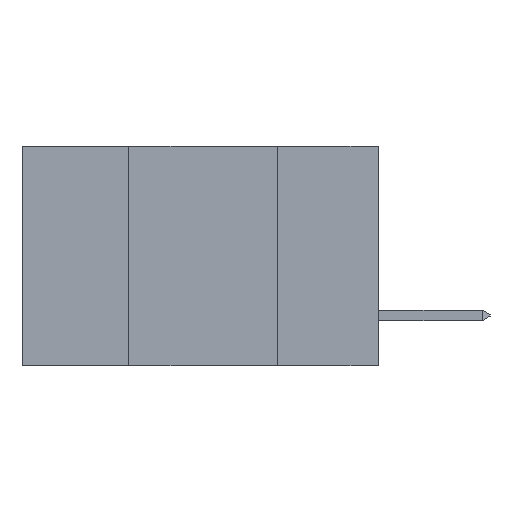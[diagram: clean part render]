
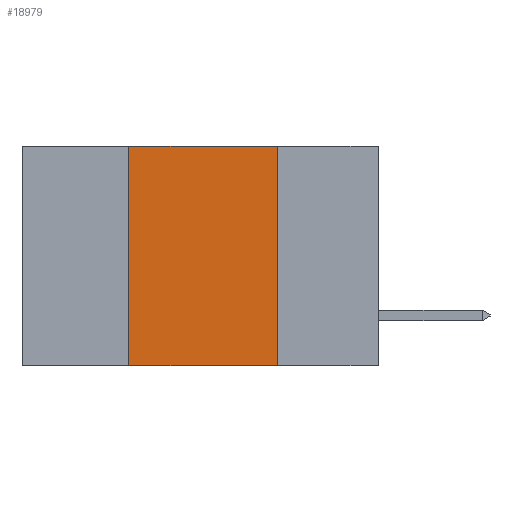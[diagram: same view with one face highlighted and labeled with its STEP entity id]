
A CAD part, left-side view. The second image highlights one B-rep face of the part: STEP entity #18979.
In plain terms, the highlighted planar face has unit normal (-1, 0, 0).
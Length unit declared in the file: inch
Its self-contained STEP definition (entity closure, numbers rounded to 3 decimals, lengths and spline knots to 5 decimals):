
#715 = EDGE_LOOP ( 'NONE', ( #17056, #18453, #7615, #10102 ) ) ;
#2209 = EDGE_CURVE ( 'NONE', #14121, #18918, #9257, .T. ) ;
#2323 = DIRECTION ( 'NONE',  ( 0., 0., -1. ) ) ;
#2471 = VERTEX_POINT ( 'NONE', #14462 ) ;
#2641 = LINE ( 'NONE', #3035, #10462 ) ;
#2938 = FACE_OUTER_BOUND ( 'NONE', #715, .T. ) ;
#3035 = CARTESIAN_POINT ( 'NONE',  ( 0., 0.42, 0. ) ) ;
#3859 = EDGE_CURVE ( 'NONE', #4077, #18918, #12831, .T. ) ;
#4077 = VERTEX_POINT ( 'NONE', #9818 ) ;
#4919 = DIRECTION ( 'NONE',  ( 0., -1., 0. ) ) ;
#5642 = EDGE_CURVE ( 'NONE', #2471, #4077, #7486, .T. ) ;
#6880 = CARTESIAN_POINT ( 'NONE',  ( 0., 0.42, -0.37 ) ) ;
#7486 = LINE ( 'NONE', #8345, #10432 ) ;
#7615 = ORIENTED_EDGE ( 'NONE', *, *, #13071, .F. ) ;
#8196 = PLANE ( 'NONE',  #12743 ) ;
#8345 = CARTESIAN_POINT ( 'NONE',  ( 0., 0.6, 0. ) ) ;
#8749 = DIRECTION ( 'NONE',  ( 0., -1., 0. ) ) ;
#9257 = LINE ( 'NONE', #16493, #17141 ) ;
#9818 = CARTESIAN_POINT ( 'NONE',  ( 0., 0.17, 0. ) ) ;
#10102 = ORIENTED_EDGE ( 'NONE', *, *, #2209, .T. ) ;
#10432 = VECTOR ( 'NONE', #8749, 39.37008 ) ;
#10462 = VECTOR ( 'NONE', #14813, 39.37008 ) ;
#11138 = DIRECTION ( 'NONE',  ( 1., 0., 0. ) ) ;
#12743 = AXIS2_PLACEMENT_3D ( 'NONE', #18533, #11138, #2323 ) ;
#12831 = LINE ( 'NONE', #16136, #16797 ) ;
#13071 = EDGE_CURVE ( 'NONE', #14121, #2471, #2641, .T. ) ;
#13920 = CARTESIAN_POINT ( 'NONE',  ( 0., 0.17, -0.37 ) ) ;
#14121 = VERTEX_POINT ( 'NONE', #6880 ) ;
#14462 = CARTESIAN_POINT ( 'NONE',  ( 0., 0.42, 0. ) ) ;
#14813 = DIRECTION ( 'NONE',  ( 0., 0., 1. ) ) ;
#16042 = DIRECTION ( 'NONE',  ( 0., 0., -1. ) ) ;
#16136 = CARTESIAN_POINT ( 'NONE',  ( 0., 0.17, 0. ) ) ;
#16493 = CARTESIAN_POINT ( 'NONE',  ( 0., 0.6, -0.37 ) ) ;
#16797 = VECTOR ( 'NONE', #16042, 39.37008 ) ;
#17056 = ORIENTED_EDGE ( 'NONE', *, *, #3859, .F. ) ;
#17141 = VECTOR ( 'NONE', #4919, 39.37008 ) ;
#18453 = ORIENTED_EDGE ( 'NONE', *, *, #5642, .F. ) ;
#18533 = CARTESIAN_POINT ( 'NONE',  ( 0., 0.6, 0. ) ) ;
#18918 = VERTEX_POINT ( 'NONE', #13920 ) ;
#18979 = ADVANCED_FACE ( 'NONE', ( #2938 ), #8196, .F. ) ;
